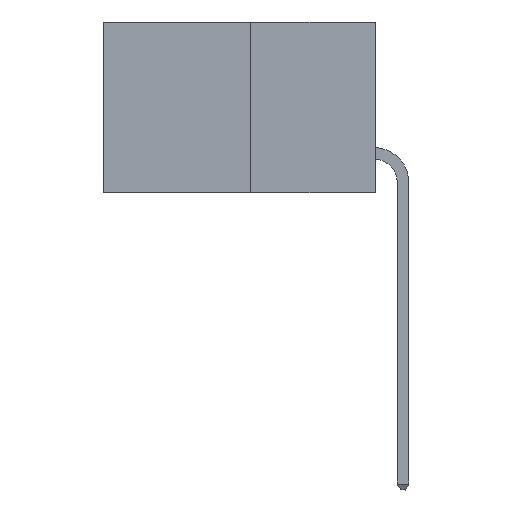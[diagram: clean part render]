
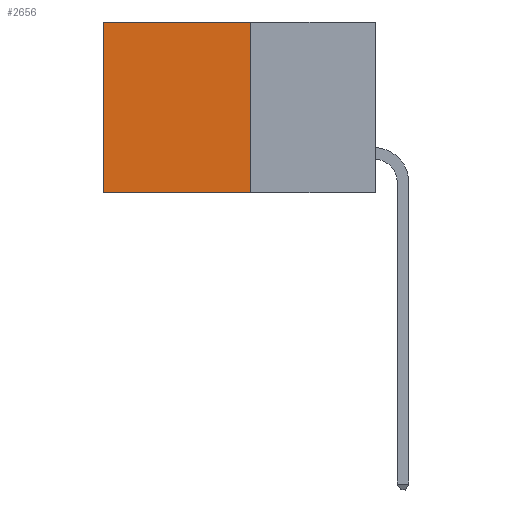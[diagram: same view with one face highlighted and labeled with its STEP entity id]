
A CAD part, left-side view. The second image highlights one B-rep face of the part: STEP entity #2656.
In plain terms, the highlighted planar face has unit normal (-1, 0, 0).
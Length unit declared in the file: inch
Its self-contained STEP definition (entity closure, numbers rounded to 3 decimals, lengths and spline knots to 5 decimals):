
#419 = DIRECTION ( 'NONE',  ( 0., 0., -1. ) ) ;
#1637 = ORIENTED_EDGE ( 'NONE', *, *, #15994, .T. ) ;
#1760 = VECTOR ( 'NONE', #13513, 39.37008 ) ;
#2656 = ADVANCED_FACE ( 'NONE', ( #11637 ), #2968, .F. ) ;
#2823 = CARTESIAN_POINT ( 'NONE',  ( 0.277, 0.27, -0.37 ) ) ;
#2968 = PLANE ( 'NONE',  #10097 ) ;
#3434 = CARTESIAN_POINT ( 'NONE',  ( 0.277, 0.59, 0. ) ) ;
#3509 = LINE ( 'NONE', #4103, #10401 ) ;
#4015 = LINE ( 'NONE', #6287, #10934 ) ;
#4103 = CARTESIAN_POINT ( 'NONE',  ( 0.277, 0.27, 0. ) ) ;
#4202 = DIRECTION ( 'NONE',  ( 0., 0., -1. ) ) ;
#4239 = EDGE_CURVE ( 'NONE', #14654, #6285, #16479, .T. ) ;
#5036 = CARTESIAN_POINT ( 'NONE',  ( 0.277, 0.59, -0.37 ) ) ;
#5478 = DIRECTION ( 'NONE',  ( 0., 1., 0. ) ) ;
#6285 = VERTEX_POINT ( 'NONE', #5036 ) ;
#6287 = CARTESIAN_POINT ( 'NONE',  ( 0.277, 0.59, -0.37 ) ) ;
#7457 = VECTOR ( 'NONE', #4202, 39.37008 ) ;
#8064 = CARTESIAN_POINT ( 'NONE',  ( 0.277, 0.27, 0. ) ) ;
#8278 = CARTESIAN_POINT ( 'NONE',  ( 0.277, 0.27, -0.37 ) ) ;
#8592 = EDGE_CURVE ( 'NONE', #10296, #14654, #11147, .T. ) ;
#9590 = EDGE_LOOP ( 'NONE', ( #1637, #11303, #15947, #11342 ) ) ;
#9897 = CARTESIAN_POINT ( 'NONE',  ( 0.277, 0.27, -0.37 ) ) ;
#10097 = AXIS2_PLACEMENT_3D ( 'NONE', #8278, #16280, #419 ) ;
#10296 = VERTEX_POINT ( 'NONE', #8064 ) ;
#10401 = VECTOR ( 'NONE', #5478, 39.37008 ) ;
#10934 = VECTOR ( 'NONE', #13176, 39.37008 ) ;
#11147 = LINE ( 'NONE', #2823, #7457 ) ;
#11303 = ORIENTED_EDGE ( 'NONE', *, *, #4239, .F. ) ;
#11342 = ORIENTED_EDGE ( 'NONE', *, *, #12860, .T. ) ;
#11637 = FACE_OUTER_BOUND ( 'NONE', #9590, .T. ) ;
#11790 = CARTESIAN_POINT ( 'NONE',  ( 0.277, 0.27, -0.37 ) ) ;
#11943 = VERTEX_POINT ( 'NONE', #3434 ) ;
#12860 = EDGE_CURVE ( 'NONE', #10296, #11943, #3509, .T. ) ;
#13176 = DIRECTION ( 'NONE',  ( 0., 0., -1. ) ) ;
#13513 = DIRECTION ( 'NONE',  ( 0., 1., 0. ) ) ;
#14654 = VERTEX_POINT ( 'NONE', #11790 ) ;
#15947 = ORIENTED_EDGE ( 'NONE', *, *, #8592, .F. ) ;
#15994 = EDGE_CURVE ( 'NONE', #11943, #6285, #4015, .T. ) ;
#16280 = DIRECTION ( 'NONE',  ( 1., 0., 0. ) ) ;
#16479 = LINE ( 'NONE', #9897, #1760 ) ;
